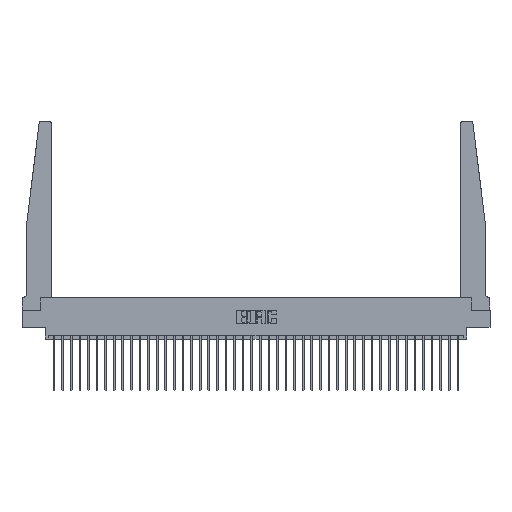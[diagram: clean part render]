
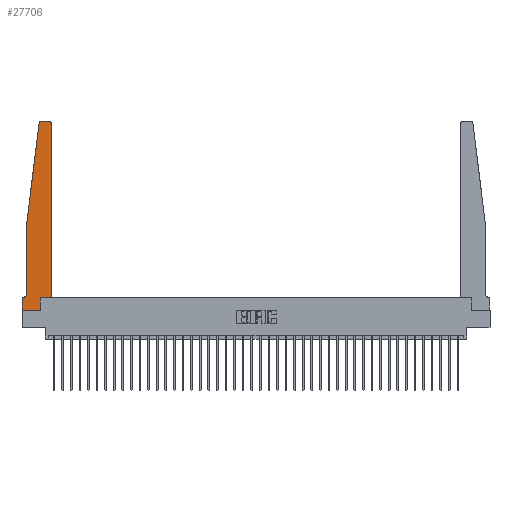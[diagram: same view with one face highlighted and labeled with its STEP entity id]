
A CAD part, top view. The second image highlights one B-rep face of the part: STEP entity #27706.
In plain terms, the highlighted planar face has unit normal (0, 0, 1).
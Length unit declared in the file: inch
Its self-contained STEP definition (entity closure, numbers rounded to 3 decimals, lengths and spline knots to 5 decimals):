
#218 = CARTESIAN_POINT ( 'NONE',  ( 0., 0.1875, 0.37 ) ) ;
#376 = CARTESIAN_POINT ( 'NONE',  ( 0.065, 0.2375, 0.37 ) ) ;
#1001 = VERTEX_POINT ( 'NONE', #21639 ) ;
#1265 = EDGE_CURVE ( 'NONE', #16077, #32490, #20132, .T. ) ;
#1563 = EDGE_CURVE ( 'NONE', #1001, #35656, #16128, .T. ) ;
#2185 = EDGE_CURVE ( 'NONE', #19320, #26393, #15116, .T. ) ;
#2892 = DIRECTION ( 'NONE',  ( 0., 0., 1. ) ) ;
#3136 = ORIENTED_EDGE ( 'NONE', *, *, #1563, .T. ) ;
#3581 = VECTOR ( 'NONE', #31280, 39.37008 ) ;
#3935 = ORIENTED_EDGE ( 'NONE', *, *, #2185, .T. ) ;
#4137 = DIRECTION ( 'NONE',  ( 1., 0., 0. ) ) ;
#5658 = LINE ( 'NONE', #22228, #35808 ) ;
#6743 = CARTESIAN_POINT ( 'NONE',  ( 0.395, 2.75, 0.37 ) ) ;
#6954 = PLANE ( 'NONE',  #27522 ) ;
#7226 = EDGE_LOOP ( 'NONE', ( #11093, #18557, #3136, #10658, #31267, #24952, #3935, #19121, #10908, #18460, #23423, #16314 ) ) ;
#8314 = CARTESIAN_POINT ( 'NONE',  ( 0.395, 2.72, 0.37 ) ) ;
#9757 = VERTEX_POINT ( 'NONE', #12480 ) ;
#9943 = CARTESIAN_POINT ( 'NONE',  ( 0.27653, 2.72, 0.37 ) ) ;
#10151 = AXIS2_PLACEMENT_3D ( 'NONE', #8314, #2892, #25068 ) ;
#10269 = EDGE_CURVE ( 'NONE', #32490, #19320, #5658, .T. ) ;
#10331 = DIRECTION ( 'NONE',  ( 1., 0., 0. ) ) ;
#10658 = ORIENTED_EDGE ( 'NONE', *, *, #31039, .T. ) ;
#10874 = CARTESIAN_POINT ( 'NONE',  ( 0.425, 0.18, 0.37 ) ) ;
#10908 = ORIENTED_EDGE ( 'NONE', *, *, #16069, .T. ) ;
#11093 = ORIENTED_EDGE ( 'NONE', *, *, #22295, .T. ) ;
#12223 = CARTESIAN_POINT ( 'NONE',  ( 0., 0., 0.37 ) ) ;
#12480 = CARTESIAN_POINT ( 'NONE',  ( 0.425, 0.18, 0.37 ) ) ;
#12580 = AXIS2_PLACEMENT_3D ( 'NONE', #9943, #18314, #4137 ) ;
#13430 = LINE ( 'NONE', #10874, #17859 ) ;
#13583 = CARTESIAN_POINT ( 'NONE',  ( 0.065, 1.25, 0.37 ) ) ;
#13643 = LINE ( 'NONE', #16367, #33899 ) ;
#13653 = CARTESIAN_POINT ( 'NONE',  ( 0.2605, 0.18, 0.37 ) ) ;
#13978 = CARTESIAN_POINT ( 'NONE',  ( 0.425, 0.18, 0.37 ) ) ;
#14171 = CARTESIAN_POINT ( 'NONE',  ( 0.015, 0.2375, 0.37 ) ) ;
#14741 = VERTEX_POINT ( 'NONE', #17462 ) ;
#14893 = CIRCLE ( 'NONE', #12580, 0.03 ) ;
#15116 = LINE ( 'NONE', #20015, #3581 ) ;
#15318 = EDGE_CURVE ( 'NONE', #15794, #1001, #14893, .T. ) ;
#15794 = VERTEX_POINT ( 'NONE', #34389 ) ;
#16069 = EDGE_CURVE ( 'NONE', #34377, #14741, #24216, .T. ) ;
#16077 = VERTEX_POINT ( 'NONE', #376 ) ;
#16128 = LINE ( 'NONE', #13583, #28583 ) ;
#16314 = ORIENTED_EDGE ( 'NONE', *, *, #31826, .T. ) ;
#16367 = CARTESIAN_POINT ( 'NONE',  ( 0., 0., 0.37 ) ) ;
#16406 = EDGE_CURVE ( 'NONE', #14741, #9757, #13430, .T. ) ;
#16597 = EDGE_CURVE ( 'NONE', #9757, #18047, #28314, .T. ) ;
#17462 = CARTESIAN_POINT ( 'NONE',  ( 0.2605, 0.18, 0.37 ) ) ;
#17859 = VECTOR ( 'NONE', #10331, 39.37008 ) ;
#18047 = VERTEX_POINT ( 'NONE', #20489 ) ;
#18314 = DIRECTION ( 'NONE',  ( 0., 0., 1. ) ) ;
#18406 = VECTOR ( 'NONE', #24755, 39.37008 ) ;
#18460 = ORIENTED_EDGE ( 'NONE', *, *, #16406, .T. ) ;
#18557 = ORIENTED_EDGE ( 'NONE', *, *, #15318, .T. ) ;
#19037 = DIRECTION ( 'NONE',  ( -0.122, -0.992, 0. ) ) ;
#19121 = ORIENTED_EDGE ( 'NONE', *, *, #30114, .T. ) ;
#19320 = VERTEX_POINT ( 'NONE', #218 ) ;
#19421 = DIRECTION ( 'NONE',  ( 0., 1., 0. ) ) ;
#20015 = CARTESIAN_POINT ( 'NONE',  ( 0., 0., 0.37 ) ) ;
#20132 = CIRCLE ( 'NONE', #31819, 0.05 ) ;
#20179 = VECTOR ( 'NONE', #19421, 39.37008 ) ;
#20489 = CARTESIAN_POINT ( 'NONE',  ( 0.425, 2.72, 0.37 ) ) ;
#21639 = CARTESIAN_POINT ( 'NONE',  ( 0.24675, 2.72367, 0.37 ) ) ;
#22228 = CARTESIAN_POINT ( 'NONE',  ( 0.065, 0.1875, 0.37 ) ) ;
#22295 = EDGE_CURVE ( 'NONE', #28348, #15794, #30862, .T. ) ;
#22352 = DIRECTION ( 'NONE',  ( -1., 0., 0. ) ) ;
#23152 = CARTESIAN_POINT ( 'NONE',  ( 0., 0.1875, 0.37 ) ) ;
#23423 = ORIENTED_EDGE ( 'NONE', *, *, #16597, .T. ) ;
#24216 = LINE ( 'NONE', #13653, #18406 ) ;
#24480 = CARTESIAN_POINT ( 'NONE',  ( 0.065, 1.25, 0.37 ) ) ;
#24657 = LINE ( 'NONE', #24480, #31007 ) ;
#24742 = DIRECTION ( 'NONE',  ( 1., 0., 0. ) ) ;
#24755 = DIRECTION ( 'NONE',  ( 0., 1., 0. ) ) ;
#24952 = ORIENTED_EDGE ( 'NONE', *, *, #10269, .T. ) ;
#25068 = DIRECTION ( 'NONE',  ( 1., 0., 0. ) ) ;
#25840 = CIRCLE ( 'NONE', #10151, 0.03 ) ;
#26393 = VERTEX_POINT ( 'NONE', #12223 ) ;
#26435 = CARTESIAN_POINT ( 'NONE',  ( 0.065, 1.25, 0.37 ) ) ;
#26782 = VECTOR ( 'NONE', #22352, 39.37008 ) ;
#27316 = DIRECTION ( 'NONE',  ( -1., 0., 0. ) ) ;
#27522 = AXIS2_PLACEMENT_3D ( 'NONE', #23152, #32038, #34948 ) ;
#27706 = ADVANCED_FACE ( 'NONE', ( #29319 ), #6954, .T. ) ;
#28314 = LINE ( 'NONE', #13978, #20179 ) ;
#28348 = VERTEX_POINT ( 'NONE', #6743 ) ;
#28583 = VECTOR ( 'NONE', #19037, 39.37008 ) ;
#29319 = FACE_OUTER_BOUND ( 'NONE', #7226, .T. ) ;
#30114 = EDGE_CURVE ( 'NONE', #26393, #34377, #13643, .T. ) ;
#30862 = LINE ( 'NONE', #31384, #26782 ) ;
#31007 = VECTOR ( 'NONE', #35544, 39.37008 ) ;
#31039 = EDGE_CURVE ( 'NONE', #35656, #16077, #24657, .T. ) ;
#31048 = DIRECTION ( 'NONE',  ( 0., 0., -1. ) ) ;
#31267 = ORIENTED_EDGE ( 'NONE', *, *, #1265, .T. ) ;
#31280 = DIRECTION ( 'NONE',  ( 0., -1., 0. ) ) ;
#31384 = CARTESIAN_POINT ( 'NONE',  ( 0.25, 2.75, 0.37 ) ) ;
#31819 = AXIS2_PLACEMENT_3D ( 'NONE', #14171, #31048, #34325 ) ;
#31826 = EDGE_CURVE ( 'NONE', #18047, #28348, #25840, .T. ) ;
#32038 = DIRECTION ( 'NONE',  ( 0., 0., 1. ) ) ;
#32490 = VERTEX_POINT ( 'NONE', #34592 ) ;
#33091 = CARTESIAN_POINT ( 'NONE',  ( 0.2605, 0., 0.37 ) ) ;
#33899 = VECTOR ( 'NONE', #24742, 39.37008 ) ;
#34325 = DIRECTION ( 'NONE',  ( -1., 0., 0. ) ) ;
#34377 = VERTEX_POINT ( 'NONE', #33091 ) ;
#34389 = CARTESIAN_POINT ( 'NONE',  ( 0.27653, 2.75, 0.37 ) ) ;
#34592 = CARTESIAN_POINT ( 'NONE',  ( 0.015, 0.1875, 0.37 ) ) ;
#34948 = DIRECTION ( 'NONE',  ( 1., 0., 0. ) ) ;
#35544 = DIRECTION ( 'NONE',  ( 0., -1., 0. ) ) ;
#35656 = VERTEX_POINT ( 'NONE', #26435 ) ;
#35808 = VECTOR ( 'NONE', #27316, 39.37008 ) ;
